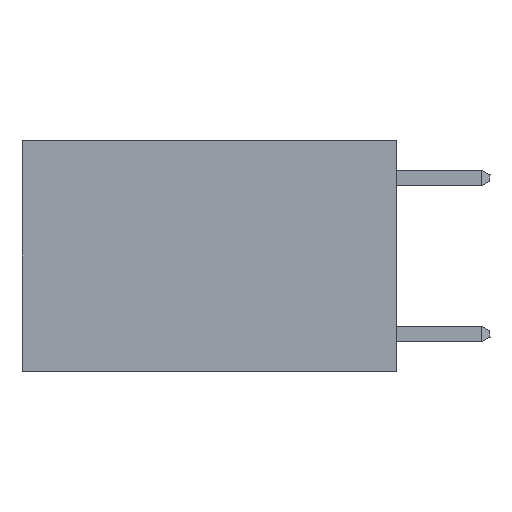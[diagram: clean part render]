
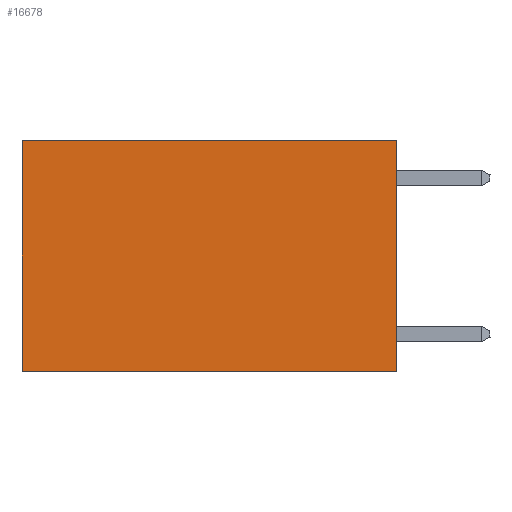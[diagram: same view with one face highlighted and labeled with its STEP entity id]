
A CAD part, left-side view. The second image highlights one B-rep face of the part: STEP entity #16678.
In plain terms, the highlighted planar face has unit normal (-1, 0, 0).
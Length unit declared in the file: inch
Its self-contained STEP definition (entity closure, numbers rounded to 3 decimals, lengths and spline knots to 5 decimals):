
#764 = CARTESIAN_POINT ( 'NONE',  ( 0.2625, 0., 0. ) ) ;
#1140 = EDGE_CURVE ( 'NONE', #6660, #6795, #21212, .T. ) ;
#1545 = CARTESIAN_POINT ( 'NONE',  ( 0.2625, 0., -0.37 ) ) ;
#1831 = CARTESIAN_POINT ( 'NONE',  ( 0.2625, 0., 0. ) ) ;
#2511 = CARTESIAN_POINT ( 'NONE',  ( 0.2625, 0., 0. ) ) ;
#3800 = CARTESIAN_POINT ( 'NONE',  ( 0.2625, 0.6, -0.37 ) ) ;
#4990 = VECTOR ( 'NONE', #20978, 39.37008 ) ;
#5318 = CARTESIAN_POINT ( 'NONE',  ( 0.2625, 0., 0. ) ) ;
#5803 = LINE ( 'NONE', #1831, #18907 ) ;
#6034 = VECTOR ( 'NONE', #22432, 39.37008 ) ;
#6397 = ORIENTED_EDGE ( 'NONE', *, *, #7743, .T. ) ;
#6660 = VERTEX_POINT ( 'NONE', #17623 ) ;
#6795 = VERTEX_POINT ( 'NONE', #3800 ) ;
#7431 = FACE_OUTER_BOUND ( 'NONE', #22736, .T. ) ;
#7743 = EDGE_CURVE ( 'NONE', #11233, #6660, #5803, .T. ) ;
#9695 = EDGE_CURVE ( 'NONE', #11233, #11792, #22209, .T. ) ;
#10776 = DIRECTION ( 'NONE',  ( 1., 0., 0. ) ) ;
#11233 = VERTEX_POINT ( 'NONE', #2511 ) ;
#11278 = EDGE_CURVE ( 'NONE', #11792, #6795, #20902, .T. ) ;
#11792 = VERTEX_POINT ( 'NONE', #1545 ) ;
#12080 = ORIENTED_EDGE ( 'NONE', *, *, #9695, .F. ) ;
#12528 = DIRECTION ( 'NONE',  ( 0., 0., -1. ) ) ;
#12640 = PLANE ( 'NONE',  #16152 ) ;
#16152 = AXIS2_PLACEMENT_3D ( 'NONE', #5318, #10776, #12528 ) ;
#16678 = ADVANCED_FACE ( 'NONE', ( #7431 ), #12640, .F. ) ;
#17246 = CARTESIAN_POINT ( 'NONE',  ( 0.2625, 0.6, 0. ) ) ;
#17623 = CARTESIAN_POINT ( 'NONE',  ( 0.2625, 0.6, 0. ) ) ;
#18438 = VECTOR ( 'NONE', #22914, 39.37008 ) ;
#18907 = VECTOR ( 'NONE', #21883, 39.37008 ) ;
#20792 = CARTESIAN_POINT ( 'NONE',  ( 0.2625, 0., -0.37 ) ) ;
#20902 = LINE ( 'NONE', #20792, #18438 ) ;
#20978 = DIRECTION ( 'NONE',  ( 0., 0., -1. ) ) ;
#21212 = LINE ( 'NONE', #17246, #4990 ) ;
#21460 = ORIENTED_EDGE ( 'NONE', *, *, #11278, .F. ) ;
#21816 = ORIENTED_EDGE ( 'NONE', *, *, #1140, .T. ) ;
#21883 = DIRECTION ( 'NONE',  ( 0., 1., 0. ) ) ;
#22209 = LINE ( 'NONE', #764, #6034 ) ;
#22432 = DIRECTION ( 'NONE',  ( 0., 0., -1. ) ) ;
#22736 = EDGE_LOOP ( 'NONE', ( #21816, #21460, #12080, #6397 ) ) ;
#22914 = DIRECTION ( 'NONE',  ( 0., 1., 0. ) ) ;
